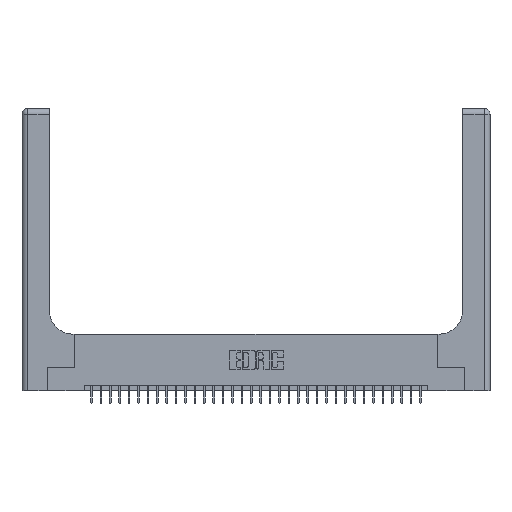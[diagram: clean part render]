
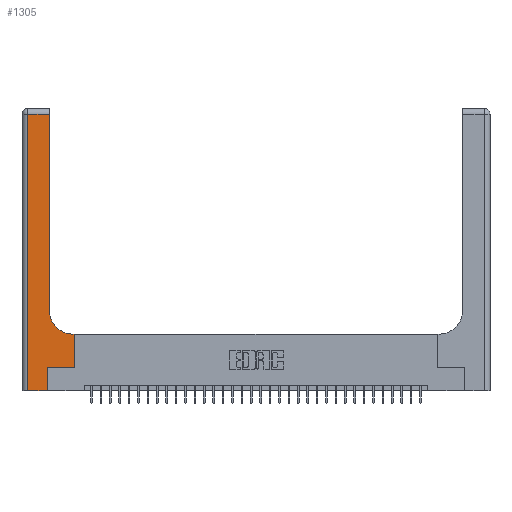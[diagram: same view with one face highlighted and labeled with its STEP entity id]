
A CAD part, top view. The second image highlights one B-rep face of the part: STEP entity #1305.
In plain terms, the highlighted planar face has unit normal (0, 0, 1).
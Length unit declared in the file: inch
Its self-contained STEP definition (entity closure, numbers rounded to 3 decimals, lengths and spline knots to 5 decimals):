
#137 = VERTEX_POINT ( 'NONE', #16977 ) ;
#220 = CARTESIAN_POINT ( 'NONE',  ( 0., 3., 0.37 ) ) ;
#749 = LINE ( 'NONE', #10635, #1504 ) ;
#1305 = ADVANCED_FACE ( 'NONE', ( #13409 ), #23992, .F. ) ;
#1469 = CARTESIAN_POINT ( 'NONE',  ( 0.269, 0.25, 0.37 ) ) ;
#1504 = VECTOR ( 'NONE', #21224, 39.37008 ) ;
#1653 = LINE ( 'NONE', #1469, #23165 ) ;
#2013 = DIRECTION ( 'NONE',  ( 1., 0., 0. ) ) ;
#2977 = VECTOR ( 'NONE', #33888, 39.37008 ) ;
#3975 = LINE ( 'NONE', #14194, #15652 ) ;
#5353 = CARTESIAN_POINT ( 'NONE',  ( 0.5415, 0.85, 0.37 ) ) ;
#6353 = VERTEX_POINT ( 'NONE', #20797 ) ;
#6796 = CARTESIAN_POINT ( 'NONE',  ( 0.5585, 0.25, 0.37 ) ) ;
#7430 = DIRECTION ( 'NONE',  ( 0., 0., -1. ) ) ;
#8057 = EDGE_CURVE ( 'NONE', #34285, #14463, #17556, .T. ) ;
#9321 = CARTESIAN_POINT ( 'NONE',  ( 0.5585, 0.6, 0.37 ) ) ;
#10437 = CARTESIAN_POINT ( 'NONE',  ( 0.269, 0., 0.37 ) ) ;
#10635 = CARTESIAN_POINT ( 'NONE',  ( 0.06, 3., 0.37 ) ) ;
#10782 = EDGE_CURVE ( 'NONE', #14463, #17649, #12491, .T. ) ;
#11302 = DIRECTION ( 'NONE',  ( -1., 0., 0. ) ) ;
#11537 = CARTESIAN_POINT ( 'NONE',  ( 0.06, 0., 0.37 ) ) ;
#12491 = LINE ( 'NONE', #20971, #2977 ) ;
#13409 = FACE_OUTER_BOUND ( 'NONE', #26034, .T. ) ;
#14005 = CARTESIAN_POINT ( 'NONE',  ( 0.5585, 0.25, 0.37 ) ) ;
#14194 = CARTESIAN_POINT ( 'NONE',  ( 0.2915, 3., 0.37 ) ) ;
#14418 = ORIENTED_EDGE ( 'NONE', *, *, #32369, .T. ) ;
#14463 = VERTEX_POINT ( 'NONE', #9321 ) ;
#14554 = DIRECTION ( 'NONE',  ( 0., 1., 0. ) ) ;
#14557 = VECTOR ( 'NONE', #2013, 39.37008 ) ;
#15015 = VECTOR ( 'NONE', #16461, 39.37008 ) ;
#15652 = VECTOR ( 'NONE', #14554, 39.37008 ) ;
#15833 = VERTEX_POINT ( 'NONE', #16119 ) ;
#16119 = CARTESIAN_POINT ( 'NONE',  ( 0.2915, 2.94, 0.37 ) ) ;
#16341 = CARTESIAN_POINT ( 'NONE',  ( 0., 2.94, 0.37 ) ) ;
#16461 = DIRECTION ( 'NONE',  ( 0., 1., 0. ) ) ;
#16977 = CARTESIAN_POINT ( 'NONE',  ( 0.2915, 0.85, 0.37 ) ) ;
#17556 = LINE ( 'NONE', #6796, #29534 ) ;
#17649 = VERTEX_POINT ( 'NONE', #30791 ) ;
#19039 = VERTEX_POINT ( 'NONE', #11537 ) ;
#19692 = DIRECTION ( 'NONE',  ( 1., 0., 0. ) ) ;
#20449 = ORIENTED_EDGE ( 'NONE', *, *, #25780, .T. ) ;
#20797 = CARTESIAN_POINT ( 'NONE',  ( 0.269, 0.25, 0.37 ) ) ;
#20930 = CARTESIAN_POINT ( 'NONE',  ( 0.06, 2.94, 0.37 ) ) ;
#20971 = CARTESIAN_POINT ( 'NONE',  ( 0.2915, 0.6, 0.37 ) ) ;
#21105 = ORIENTED_EDGE ( 'NONE', *, *, #10782, .T. ) ;
#21224 = DIRECTION ( 'NONE',  ( 0., -1., 0. ) ) ;
#21384 = DIRECTION ( 'NONE',  ( 0., 0., -1. ) ) ;
#23165 = VECTOR ( 'NONE', #19692, 39.37008 ) ;
#23992 = PLANE ( 'NONE',  #27059 ) ;
#24480 = LINE ( 'NONE', #16341, #27237 ) ;
#24651 = EDGE_CURVE ( 'NONE', #25386, #19039, #749, .T. ) ;
#24876 = ORIENTED_EDGE ( 'NONE', *, *, #29170, .T. ) ;
#24971 = ORIENTED_EDGE ( 'NONE', *, *, #24651, .T. ) ;
#25094 = CIRCLE ( 'NONE', #28468, 0.25 ) ;
#25386 = VERTEX_POINT ( 'NONE', #20930 ) ;
#25780 = EDGE_CURVE ( 'NONE', #6353, #34285, #1653, .T. ) ;
#25798 = LINE ( 'NONE', #28607, #14557 ) ;
#26034 = EDGE_LOOP ( 'NONE', ( #14418, #28370, #24971, #27668, #24876, #20449, #32218, #21105, #27254 ) ) ;
#27059 = AXIS2_PLACEMENT_3D ( 'NONE', #220, #21384, #32040 ) ;
#27237 = VECTOR ( 'NONE', #11302, 39.37008 ) ;
#27254 = ORIENTED_EDGE ( 'NONE', *, *, #33019, .T. ) ;
#27613 = LINE ( 'NONE', #29742, #15015 ) ;
#27668 = ORIENTED_EDGE ( 'NONE', *, *, #32765, .T. ) ;
#27735 = EDGE_CURVE ( 'NONE', #15833, #25386, #24480, .T. ) ;
#28197 = DIRECTION ( 'NONE',  ( 0., 1., 0. ) ) ;
#28370 = ORIENTED_EDGE ( 'NONE', *, *, #27735, .T. ) ;
#28468 = AXIS2_PLACEMENT_3D ( 'NONE', #5353, #7430, #33696 ) ;
#28607 = CARTESIAN_POINT ( 'NONE',  ( 0., 0., 0.37 ) ) ;
#29170 = EDGE_CURVE ( 'NONE', #31797, #6353, #27613, .T. ) ;
#29534 = VECTOR ( 'NONE', #28197, 39.37008 ) ;
#29742 = CARTESIAN_POINT ( 'NONE',  ( 0.269, 0., 0.37 ) ) ;
#30791 = CARTESIAN_POINT ( 'NONE',  ( 0.5415, 0.6, 0.37 ) ) ;
#31797 = VERTEX_POINT ( 'NONE', #10437 ) ;
#32040 = DIRECTION ( 'NONE',  ( -1., 0., 0. ) ) ;
#32218 = ORIENTED_EDGE ( 'NONE', *, *, #8057, .T. ) ;
#32369 = EDGE_CURVE ( 'NONE', #137, #15833, #3975, .T. ) ;
#32765 = EDGE_CURVE ( 'NONE', #19039, #31797, #25798, .T. ) ;
#33019 = EDGE_CURVE ( 'NONE', #17649, #137, #25094, .T. ) ;
#33696 = DIRECTION ( 'NONE',  ( 1., 0., 0. ) ) ;
#33888 = DIRECTION ( 'NONE',  ( -1., 0., 0. ) ) ;
#34285 = VERTEX_POINT ( 'NONE', #14005 ) ;
